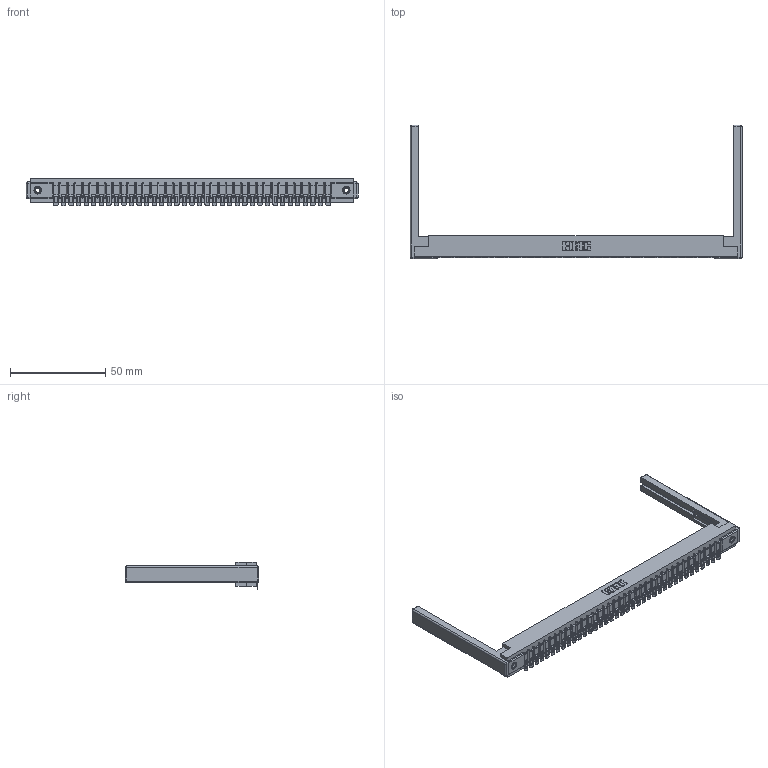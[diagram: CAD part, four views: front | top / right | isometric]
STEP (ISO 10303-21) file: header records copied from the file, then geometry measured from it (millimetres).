
FILE_DESCRIPTION (( 'STEP AP203' ), '1' );
FILE_NAME ('307-037-554-168.STEP', '2019-09-05T08:42:19', ( '' ), ( '' ), 'SwSTEP 2.0', 'SolidWorks 2016', '' );
FILE_SCHEMA (( 'CONFIG_CONTROL_DESIGN' ));
Length unit declared in the file: inch
Products named in the file (5): 307-037-554-168; 345-250-001_345-250-001-102; 307-220-068; 307-290-002_554; 307 Part_.156 Dia Mounting Holes
Assembly tree (42 placements, depth 2):
  307-037-554-168
    307 Part_.156 Dia Mounting Holes
    307-290-002_554  x37
    307-220-068  x2
    345-250-001_345-250-001-102  x2
Bounding box: 174.04 x 69.98 x 14.52 mm (x, y, z)
Volume: 22978.2 mm3; surface area: 27381.8 mm2
Topology: 42 solids, 42 shells, 3307 faces, 10074 edges, 6592 vertices
Faces by surface type: plane 1860, cylinder 1347, sphere 84, cone 12, torus 4
Entity records: 36060 total; most frequent: CARTESIAN_POINT 6047, ORIENTED_EDGE 6026, DIRECTION 5901, EDGE_CURVE 3013, LINE 2297, VECTOR 2297, VERTEX_POINT 1948, AXIS2_PLACEMENT_3D 1802
